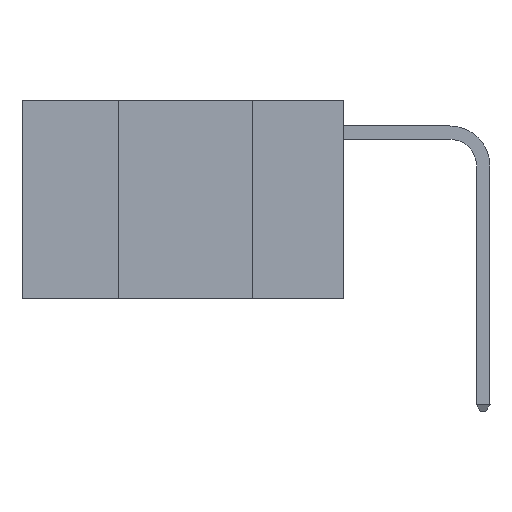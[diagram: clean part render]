
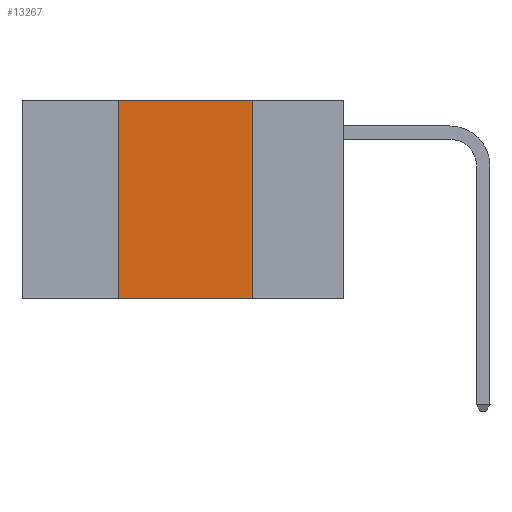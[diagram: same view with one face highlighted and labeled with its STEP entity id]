
A CAD part, left-side view. The second image highlights one B-rep face of the part: STEP entity #13267.
In plain terms, the highlighted planar face has unit normal (-1, 0, 0).
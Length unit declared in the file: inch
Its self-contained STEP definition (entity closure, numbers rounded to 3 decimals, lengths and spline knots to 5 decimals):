
#359 = CARTESIAN_POINT ( 'NONE',  ( 0., 0.6, 0. ) ) ;
#1810 = VECTOR ( 'NONE', #8470, 39.37008 ) ;
#2435 = LINE ( 'NONE', #3883, #9190 ) ;
#3034 = EDGE_LOOP ( 'NONE', ( #10756, #13671, #3802, #15405 ) ) ;
#3760 = DIRECTION ( 'NONE',  ( 0., 0., -1. ) ) ;
#3802 = ORIENTED_EDGE ( 'NONE', *, *, #8758, .F. ) ;
#3883 = CARTESIAN_POINT ( 'NONE',  ( 0., 0.17, 0. ) ) ;
#3899 = VECTOR ( 'NONE', #9712, 39.37008 ) ;
#4086 = CARTESIAN_POINT ( 'NONE',  ( 0., 0.42, 0. ) ) ;
#4295 = CARTESIAN_POINT ( 'NONE',  ( 0., 0.6, -0.37 ) ) ;
#4935 = CARTESIAN_POINT ( 'NONE',  ( 0., 0.17, -0.37 ) ) ;
#5421 = LINE ( 'NONE', #359, #1810 ) ;
#7237 = VERTEX_POINT ( 'NONE', #4086 ) ;
#7371 = AXIS2_PLACEMENT_3D ( 'NONE', #10469, #11821, #3760 ) ;
#7474 = LINE ( 'NONE', #4295, #3899 ) ;
#8319 = EDGE_CURVE ( 'NONE', #12493, #12683, #2435, .T. ) ;
#8470 = DIRECTION ( 'NONE',  ( 0., -1., 0. ) ) ;
#8758 = EDGE_CURVE ( 'NONE', #15656, #7237, #15467, .T. ) ;
#9098 = PLANE ( 'NONE',  #7371 ) ;
#9190 = VECTOR ( 'NONE', #13268, 39.37008 ) ;
#9235 = EDGE_CURVE ( 'NONE', #15656, #12683, #7474, .T. ) ;
#9635 = CARTESIAN_POINT ( 'NONE',  ( 0., 0.42, -0.37 ) ) ;
#9712 = DIRECTION ( 'NONE',  ( 0., -1., 0. ) ) ;
#9795 = FACE_OUTER_BOUND ( 'NONE', #3034, .T. ) ;
#10469 = CARTESIAN_POINT ( 'NONE',  ( 0., 0.6, 0. ) ) ;
#10756 = ORIENTED_EDGE ( 'NONE', *, *, #8319, .F. ) ;
#11218 = CARTESIAN_POINT ( 'NONE',  ( 0., 0.17, 0. ) ) ;
#11499 = CARTESIAN_POINT ( 'NONE',  ( 0., 0.42, 0. ) ) ;
#11821 = DIRECTION ( 'NONE',  ( 1., 0., 0. ) ) ;
#12475 = EDGE_CURVE ( 'NONE', #7237, #12493, #5421, .T. ) ;
#12493 = VERTEX_POINT ( 'NONE', #11218 ) ;
#12683 = VERTEX_POINT ( 'NONE', #4935 ) ;
#13267 = ADVANCED_FACE ( 'NONE', ( #9795 ), #9098, .F. ) ;
#13268 = DIRECTION ( 'NONE',  ( 0., 0., -1. ) ) ;
#13671 = ORIENTED_EDGE ( 'NONE', *, *, #12475, .F. ) ;
#14134 = DIRECTION ( 'NONE',  ( 0., 0., 1. ) ) ;
#14622 = VECTOR ( 'NONE', #14134, 39.37008 ) ;
#15405 = ORIENTED_EDGE ( 'NONE', *, *, #9235, .T. ) ;
#15467 = LINE ( 'NONE', #11499, #14622 ) ;
#15656 = VERTEX_POINT ( 'NONE', #9635 ) ;
